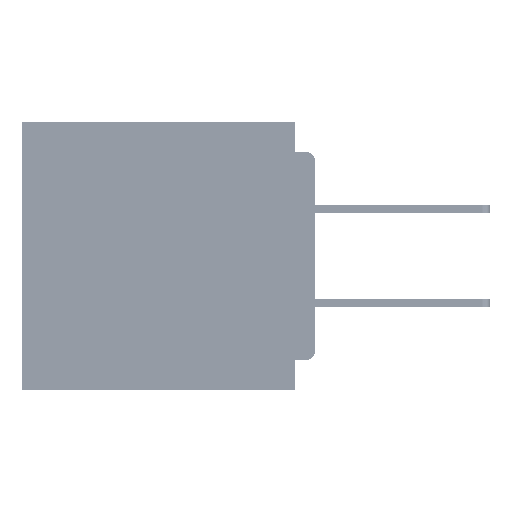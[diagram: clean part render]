
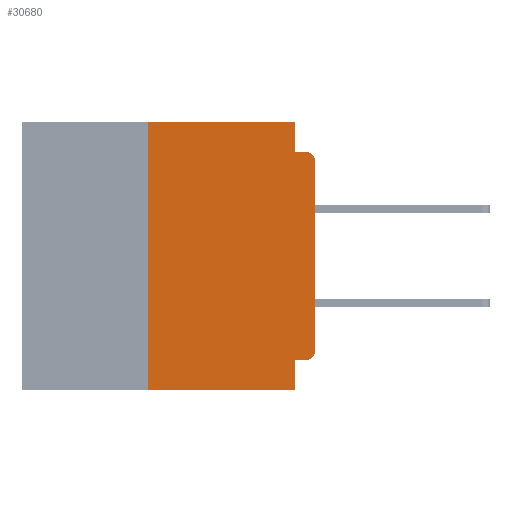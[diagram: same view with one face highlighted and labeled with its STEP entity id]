
A CAD part, left-side view. The second image highlights one B-rep face of the part: STEP entity #30680.
In plain terms, the highlighted planar face has unit normal (-1, 0, 0).
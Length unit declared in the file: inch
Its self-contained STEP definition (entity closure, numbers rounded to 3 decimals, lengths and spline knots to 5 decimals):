
#311 = ORIENTED_EDGE ( 'NONE', *, *, #67675, .F. ) ;
#911 = ORIENTED_EDGE ( 'NONE', *, *, #60466, .T. ) ;
#1424 = CARTESIAN_POINT ( 'NONE',  ( 0., 0.031, -0.4 ) ) ;
#1665 = DIRECTION ( 'NONE',  ( 0., 1., 0. ) ) ;
#4618 = DIRECTION ( 'NONE',  ( 0., 0., 1. ) ) ;
#5780 = CARTESIAN_POINT ( 'NONE',  ( 0., 0.015, -0.34 ) ) ;
#6158 = CARTESIAN_POINT ( 'NONE',  ( 0., 0.437, 0. ) ) ;
#7428 = LINE ( 'NONE', #22653, #18663 ) ;
#8066 = DIRECTION ( 'NONE',  ( 0., 0., -1. ) ) ;
#8476 = EDGE_CURVE ( 'NONE', #39762, #71169, #44062, .T. ) ;
#9177 = VERTEX_POINT ( 'NONE', #63425 ) ;
#10344 = ORIENTED_EDGE ( 'NONE', *, *, #16289, .T. ) ;
#10982 = LINE ( 'NONE', #17934, #24014 ) ;
#11319 = DIRECTION ( 'NONE',  ( 0., 0., -1. ) ) ;
#11695 = DIRECTION ( 'NONE',  ( 0., 0., -1. ) ) ;
#12178 = FACE_OUTER_BOUND ( 'NONE', #16699, .T. ) ;
#12908 = VECTOR ( 'NONE', #8066, 39.37008 ) ;
#15208 = AXIS2_PLACEMENT_3D ( 'NONE', #5780, #44453, #11319 ) ;
#15327 = CARTESIAN_POINT ( 'NONE',  ( 0., 0.25, 0. ) ) ;
#15876 = EDGE_CURVE ( 'NONE', #45618, #34367, #57489, .T. ) ;
#16289 = EDGE_CURVE ( 'NONE', #68290, #21608, #43915, .T. ) ;
#16699 = EDGE_LOOP ( 'NONE', ( #70904, #10344, #60338, #311, #58819, #60751, #911, #63018, #63364, #63650 ) ) ;
#17270 = DIRECTION ( 'NONE',  ( 0., 0., -1. ) ) ;
#17854 = VECTOR ( 'NONE', #35268, 39.37008 ) ;
#17934 = CARTESIAN_POINT ( 'NONE',  ( 0., 0.437, 0. ) ) ;
#18663 = VECTOR ( 'NONE', #17270, 39.37008 ) ;
#19331 = EDGE_CURVE ( 'NONE', #35217, #21608, #20261, .T. ) ;
#19825 = CARTESIAN_POINT ( 'NONE',  ( 0., 0.015, -0.06 ) ) ;
#20261 = LINE ( 'NONE', #47466, #34972 ) ;
#21608 = VERTEX_POINT ( 'NONE', #24294 ) ;
#22653 = CARTESIAN_POINT ( 'NONE',  ( 0., 0.031, 0. ) ) ;
#23076 = CARTESIAN_POINT ( 'NONE',  ( 0., 0., -0.06 ) ) ;
#23438 = DIRECTION ( 'NONE',  ( 0., -1., 0. ) ) ;
#23774 = CARTESIAN_POINT ( 'NONE',  ( 0., 0., -0.355 ) ) ;
#24014 = VECTOR ( 'NONE', #62029, 39.37008 ) ;
#24294 = CARTESIAN_POINT ( 'NONE',  ( 0., 0.015, -0.045 ) ) ;
#25149 = EDGE_CURVE ( 'NONE', #9177, #53345, #31230, .T. ) ;
#25422 = DIRECTION ( 'NONE',  ( 0., 0., -1. ) ) ;
#26680 = CARTESIAN_POINT ( 'NONE',  ( 0., 0.25, -0.4 ) ) ;
#27279 = EDGE_CURVE ( 'NONE', #53345, #68290, #47222, .T. ) ;
#28761 = CARTESIAN_POINT ( 'NONE',  ( 0., 0.437, -0.4 ) ) ;
#29954 = CARTESIAN_POINT ( 'NONE',  ( 0., 0., 0. ) ) ;
#30680 = ADVANCED_FACE ( 'NONE', ( #12178 ), #66577, .F. ) ;
#31230 = CIRCLE ( 'NONE', #15208, 0.015 ) ;
#33094 = CARTESIAN_POINT ( 'NONE',  ( 0., 0.031, -0.355 ) ) ;
#33752 = LINE ( 'NONE', #28761, #46633 ) ;
#34367 = VERTEX_POINT ( 'NONE', #15327 ) ;
#34907 = AXIS2_PLACEMENT_3D ( 'NONE', #19825, #58376, #25422 ) ;
#34972 = VECTOR ( 'NONE', #53000, 39.37008 ) ;
#35217 = VERTEX_POINT ( 'NONE', #66689 ) ;
#35268 = DIRECTION ( 'NONE',  ( 0., 0., 1. ) ) ;
#38796 = VERTEX_POINT ( 'NONE', #53446 ) ;
#39762 = VERTEX_POINT ( 'NONE', #33094 ) ;
#41181 = VECTOR ( 'NONE', #4618, 39.37008 ) ;
#41796 = VECTOR ( 'NONE', #1665, 39.37008 ) ;
#43915 = CIRCLE ( 'NONE', #34907, 0.015 ) ;
#44062 = LINE ( 'NONE', #46711, #12908 ) ;
#44453 = DIRECTION ( 'NONE',  ( -1., 0., 0. ) ) ;
#44817 = DIRECTION ( 'NONE',  ( 1., 0., 0. ) ) ;
#45618 = VERTEX_POINT ( 'NONE', #62970 ) ;
#46633 = VECTOR ( 'NONE', #23438, 39.37008 ) ;
#46711 = CARTESIAN_POINT ( 'NONE',  ( 0., 0.031, -0.4 ) ) ;
#47222 = LINE ( 'NONE', #29954, #17854 ) ;
#47466 = CARTESIAN_POINT ( 'NONE',  ( 0., 0., -0.045 ) ) ;
#51972 = AXIS2_PLACEMENT_3D ( 'NONE', #6158, #44817, #11695 ) ;
#53000 = DIRECTION ( 'NONE',  ( 0., -1., 0. ) ) ;
#53345 = VERTEX_POINT ( 'NONE', #66088 ) ;
#53446 = CARTESIAN_POINT ( 'NONE',  ( 0., 0.031, 0. ) ) ;
#56198 = EDGE_CURVE ( 'NONE', #9177, #39762, #58092, .T. ) ;
#57489 = LINE ( 'NONE', #26680, #41181 ) ;
#58092 = LINE ( 'NONE', #23774, #41796 ) ;
#58376 = DIRECTION ( 'NONE',  ( -1., 0., 0. ) ) ;
#58819 = ORIENTED_EDGE ( 'NONE', *, *, #71165, .F. ) ;
#60338 = ORIENTED_EDGE ( 'NONE', *, *, #19331, .F. ) ;
#60466 = EDGE_CURVE ( 'NONE', #45618, #71169, #33752, .T. ) ;
#60751 = ORIENTED_EDGE ( 'NONE', *, *, #15876, .F. ) ;
#62029 = DIRECTION ( 'NONE',  ( 0., -1., 0. ) ) ;
#62970 = CARTESIAN_POINT ( 'NONE',  ( 0., 0.25, -0.4 ) ) ;
#63018 = ORIENTED_EDGE ( 'NONE', *, *, #8476, .F. ) ;
#63364 = ORIENTED_EDGE ( 'NONE', *, *, #56198, .F. ) ;
#63425 = CARTESIAN_POINT ( 'NONE',  ( 0., 0.015, -0.355 ) ) ;
#63650 = ORIENTED_EDGE ( 'NONE', *, *, #25149, .T. ) ;
#66088 = CARTESIAN_POINT ( 'NONE',  ( 0., 0., -0.34 ) ) ;
#66577 = PLANE ( 'NONE',  #51972 ) ;
#66689 = CARTESIAN_POINT ( 'NONE',  ( 0., 0.031, -0.045 ) ) ;
#67675 = EDGE_CURVE ( 'NONE', #38796, #35217, #7428, .T. ) ;
#68290 = VERTEX_POINT ( 'NONE', #23076 ) ;
#70904 = ORIENTED_EDGE ( 'NONE', *, *, #27279, .T. ) ;
#71165 = EDGE_CURVE ( 'NONE', #34367, #38796, #10982, .T. ) ;
#71169 = VERTEX_POINT ( 'NONE', #1424 ) ;
